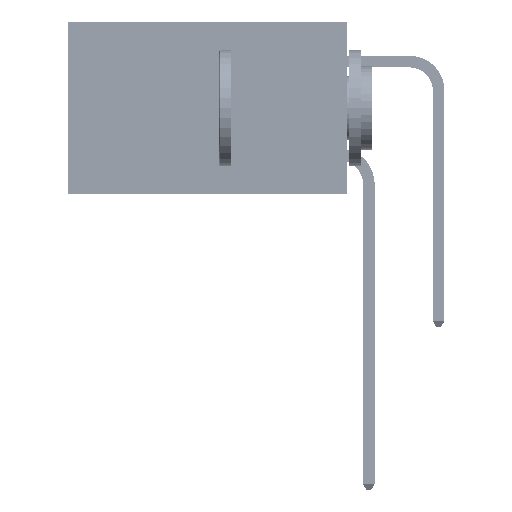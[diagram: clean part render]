
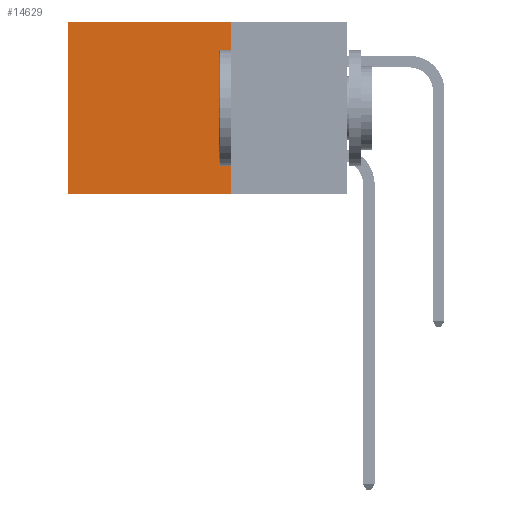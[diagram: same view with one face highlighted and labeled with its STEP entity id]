
A CAD part, left-side view. The second image highlights one B-rep face of the part: STEP entity #14629.
In plain terms, the highlighted planar face has unit normal (-1, 0, 0).
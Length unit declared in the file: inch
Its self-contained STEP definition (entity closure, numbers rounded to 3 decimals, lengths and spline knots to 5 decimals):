
#441 = CARTESIAN_POINT ( 'NONE',  ( 0.2875, 0.25, -0.37 ) ) ;
#1711 = ORIENTED_EDGE ( 'NONE', *, *, #43378, .F. ) ;
#3424 = AXIS2_PLACEMENT_3D ( 'NONE', #16860, #9177, #36398 ) ;
#3916 = VERTEX_POINT ( 'NONE', #46443 ) ;
#4405 = DIRECTION ( 'NONE',  ( 0., 1., 0. ) ) ;
#5012 = EDGE_LOOP ( 'NONE', ( #29525, #1711, #30731, #21359 ) ) ;
#7619 = EDGE_CURVE ( 'NONE', #21201, #16125, #24690, .T. ) ;
#9177 = DIRECTION ( 'NONE',  ( 1., 0., 0. ) ) ;
#11548 = VECTOR ( 'NONE', #26044, 39.37008 ) ;
#13650 = DIRECTION ( 'NONE',  ( 0., 0., -1. ) ) ;
#14629 = ADVANCED_FACE ( 'NONE', ( #14702 ), #47786, .F. ) ;
#14702 = FACE_OUTER_BOUND ( 'NONE', #5012, .T. ) ;
#14902 = VERTEX_POINT ( 'NONE', #49565 ) ;
#15579 = VECTOR ( 'NONE', #4405, 39.37008 ) ;
#16125 = VERTEX_POINT ( 'NONE', #44459 ) ;
#16860 = CARTESIAN_POINT ( 'NONE',  ( 0.2875, 0.25, 0. ) ) ;
#19327 = CARTESIAN_POINT ( 'NONE',  ( 0.2875, 0.6, 0. ) ) ;
#19419 = EDGE_CURVE ( 'NONE', #14902, #3916, #19830, .T. ) ;
#19830 = LINE ( 'NONE', #19327, #21055 ) ;
#20707 = LINE ( 'NONE', #49131, #11548 ) ;
#21055 = VECTOR ( 'NONE', #46380, 39.37008 ) ;
#21201 = VERTEX_POINT ( 'NONE', #37166 ) ;
#21359 = ORIENTED_EDGE ( 'NONE', *, *, #38826, .T. ) ;
#24690 = LINE ( 'NONE', #44651, #33795 ) ;
#26044 = DIRECTION ( 'NONE',  ( 0., 1., 0. ) ) ;
#29525 = ORIENTED_EDGE ( 'NONE', *, *, #19419, .T. ) ;
#30731 = ORIENTED_EDGE ( 'NONE', *, *, #7619, .F. ) ;
#33795 = VECTOR ( 'NONE', #13650, 39.37008 ) ;
#36398 = DIRECTION ( 'NONE',  ( 0., 0., -1. ) ) ;
#37166 = CARTESIAN_POINT ( 'NONE',  ( 0.2875, 0.25, 0. ) ) ;
#38826 = EDGE_CURVE ( 'NONE', #21201, #14902, #20707, .T. ) ;
#43378 = EDGE_CURVE ( 'NONE', #16125, #3916, #46468, .T. ) ;
#44459 = CARTESIAN_POINT ( 'NONE',  ( 0.2875, 0.25, -0.37 ) ) ;
#44651 = CARTESIAN_POINT ( 'NONE',  ( 0.2875, 0.25, 0. ) ) ;
#46380 = DIRECTION ( 'NONE',  ( 0., 0., -1. ) ) ;
#46443 = CARTESIAN_POINT ( 'NONE',  ( 0.2875, 0.6, -0.37 ) ) ;
#46468 = LINE ( 'NONE', #441, #15579 ) ;
#47786 = PLANE ( 'NONE',  #3424 ) ;
#49131 = CARTESIAN_POINT ( 'NONE',  ( 0.2875, 0.25, 0. ) ) ;
#49565 = CARTESIAN_POINT ( 'NONE',  ( 0.2875, 0.6, 0. ) ) ;
